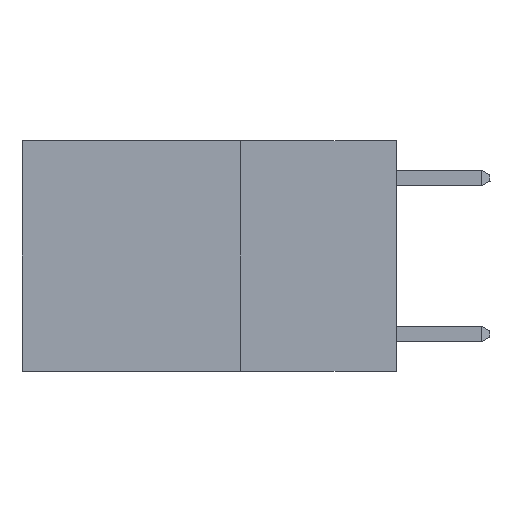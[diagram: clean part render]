
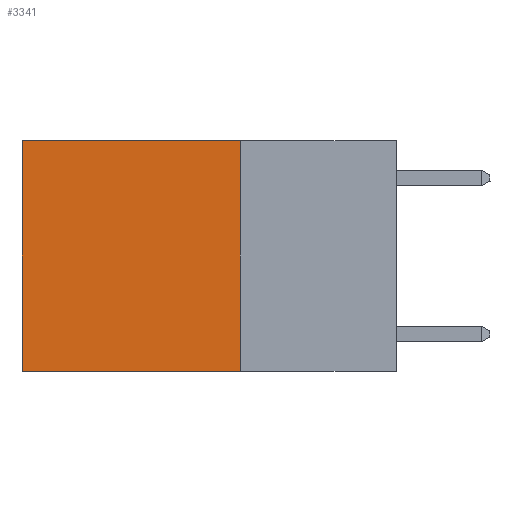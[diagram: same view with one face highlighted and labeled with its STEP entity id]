
A CAD part, left-side view. The second image highlights one B-rep face of the part: STEP entity #3341.
In plain terms, the highlighted planar face has unit normal (-1, 0, 0).
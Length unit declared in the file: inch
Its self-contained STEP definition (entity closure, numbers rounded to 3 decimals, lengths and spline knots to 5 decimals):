
#338 = DIRECTION ( 'NONE',  ( 0., 0., -1. ) ) ;
#380 = EDGE_CURVE ( 'NONE', #2877, #8057, #1746, .T. ) ;
#508 = EDGE_CURVE ( 'NONE', #4930, #2756, #2855, .T. ) ;
#532 = VECTOR ( 'NONE', #2702, 39.37008 ) ;
#1120 = PLANE ( 'NONE',  #7415 ) ;
#1337 = CARTESIAN_POINT ( 'NONE',  ( 0.2625, 0.25, 0. ) ) ;
#1604 = FACE_OUTER_BOUND ( 'NONE', #2411, .T. ) ;
#1746 = LINE ( 'NONE', #6672, #4493 ) ;
#1825 = EDGE_CURVE ( 'NONE', #2756, #8057, #5883, .T. ) ;
#2411 = EDGE_LOOP ( 'NONE', ( #5369, #6369, #6363, #5546 ) ) ;
#2702 = DIRECTION ( 'NONE',  ( 0., 0., -1. ) ) ;
#2756 = VERTEX_POINT ( 'NONE', #7326 ) ;
#2855 = LINE ( 'NONE', #7692, #532 ) ;
#2877 = VERTEX_POINT ( 'NONE', #3711 ) ;
#3098 = EDGE_CURVE ( 'NONE', #4930, #2877, #9000, .T. ) ;
#3341 = ADVANCED_FACE ( 'NONE', ( #1604 ), #1120, .F. ) ;
#3711 = CARTESIAN_POINT ( 'NONE',  ( 0.2625, 0.6, 0. ) ) ;
#3989 = CARTESIAN_POINT ( 'NONE',  ( 0.2625, 0.25, 0. ) ) ;
#4108 = DIRECTION ( 'NONE',  ( 0., 1., 0. ) ) ;
#4493 = VECTOR ( 'NONE', #338, 39.37008 ) ;
#4605 = CARTESIAN_POINT ( 'NONE',  ( 0.2625, 0.25, -0.37 ) ) ;
#4753 = CARTESIAN_POINT ( 'NONE',  ( 0.2625, 0.6, -0.37 ) ) ;
#4756 = DIRECTION ( 'NONE',  ( 1., 0., 0. ) ) ;
#4930 = VERTEX_POINT ( 'NONE', #7484 ) ;
#5369 = ORIENTED_EDGE ( 'NONE', *, *, #380, .T. ) ;
#5546 = ORIENTED_EDGE ( 'NONE', *, *, #3098, .T. ) ;
#5883 = LINE ( 'NONE', #4605, #9065 ) ;
#6363 = ORIENTED_EDGE ( 'NONE', *, *, #508, .F. ) ;
#6369 = ORIENTED_EDGE ( 'NONE', *, *, #1825, .F. ) ;
#6672 = CARTESIAN_POINT ( 'NONE',  ( 0.2625, 0.6, 0. ) ) ;
#6736 = VECTOR ( 'NONE', #4108, 39.37008 ) ;
#7326 = CARTESIAN_POINT ( 'NONE',  ( 0.2625, 0.25, -0.37 ) ) ;
#7415 = AXIS2_PLACEMENT_3D ( 'NONE', #3989, #4756, #8478 ) ;
#7484 = CARTESIAN_POINT ( 'NONE',  ( 0.2625, 0.25, 0. ) ) ;
#7692 = CARTESIAN_POINT ( 'NONE',  ( 0.2625, 0.25, 0. ) ) ;
#8057 = VERTEX_POINT ( 'NONE', #4753 ) ;
#8255 = DIRECTION ( 'NONE',  ( 0., 1., 0. ) ) ;
#8478 = DIRECTION ( 'NONE',  ( 0., 0., -1. ) ) ;
#9000 = LINE ( 'NONE', #1337, #6736 ) ;
#9065 = VECTOR ( 'NONE', #8255, 39.37008 ) ;
